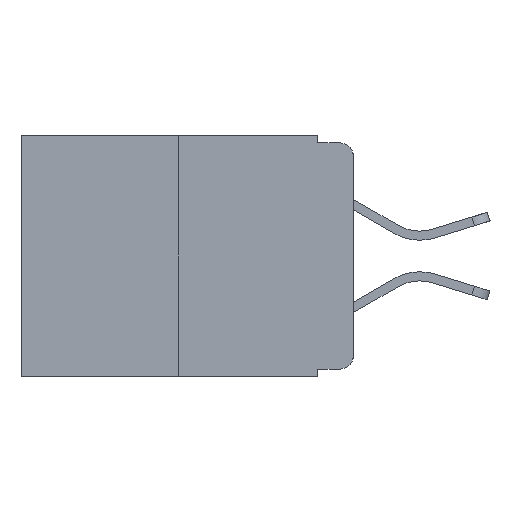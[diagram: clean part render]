
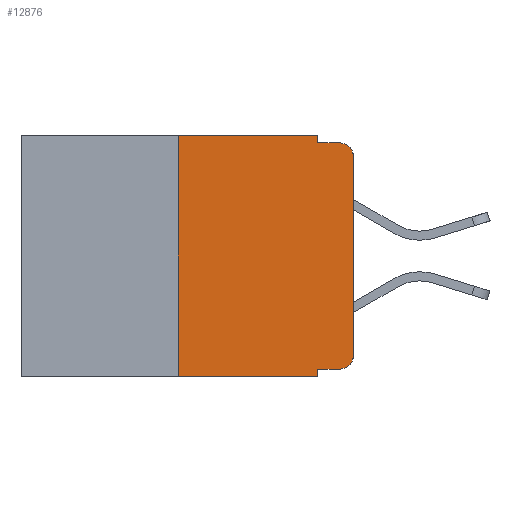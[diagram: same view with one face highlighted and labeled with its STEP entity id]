
A CAD part, left-side view. The second image highlights one B-rep face of the part: STEP entity #12876.
In plain terms, the highlighted planar face has unit normal (-1, 0, 0).
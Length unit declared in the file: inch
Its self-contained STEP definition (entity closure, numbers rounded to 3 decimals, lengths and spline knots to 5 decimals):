
#13 = DIRECTION ( 'NONE',  ( 0., 0., -1. ) ) ;
#335 = DIRECTION ( 'NONE',  ( 0., 0., -1. ) ) ;
#521 = VECTOR ( 'NONE', #4729, 39.37008 ) ;
#529 = CARTESIAN_POINT ( 'NONE',  ( 0., 0.051, -0.343 ) ) ;
#798 = LINE ( 'NONE', #15091, #11758 ) ;
#930 = LINE ( 'NONE', #16887, #11429 ) ;
#941 = CARTESIAN_POINT ( 'NONE',  ( 0., 0.25, 0. ) ) ;
#1084 = EDGE_CURVE ( 'NONE', #4803, #3712, #8154, .T. ) ;
#2283 = DIRECTION ( 'NONE',  ( -1., 0., 0. ) ) ;
#2502 = LINE ( 'NONE', #14109, #13431 ) ;
#2797 = CARTESIAN_POINT ( 'NONE',  ( 0., 0.473, 0. ) ) ;
#2988 = VERTEX_POINT ( 'NONE', #7426 ) ;
#3042 = EDGE_CURVE ( 'NONE', #4803, #16492, #13799, .T. ) ;
#3497 = CIRCLE ( 'NONE', #4543, 0.02 ) ;
#3712 = VERTEX_POINT ( 'NONE', #9028 ) ;
#4163 = CARTESIAN_POINT ( 'NONE',  ( 0., 0.02, -0.01 ) ) ;
#4246 = DIRECTION ( 'NONE',  ( 0., 0., -1. ) ) ;
#4267 = DIRECTION ( 'NONE',  ( 0., -1., 0. ) ) ;
#4543 = AXIS2_PLACEMENT_3D ( 'NONE', #8289, #17995, #9701 ) ;
#4729 = DIRECTION ( 'NONE',  ( 0., 0., 1. ) ) ;
#4803 = VERTEX_POINT ( 'NONE', #5604 ) ;
#4942 = ORIENTED_EDGE ( 'NONE', *, *, #16857, .T. ) ;
#4988 = EDGE_CURVE ( 'NONE', #12511, #10292, #11922, .T. ) ;
#5346 = LINE ( 'NONE', #14137, #6709 ) ;
#5362 = CARTESIAN_POINT ( 'NONE',  ( 0., 0.051, -0.01 ) ) ;
#5394 = ORIENTED_EDGE ( 'NONE', *, *, #1084, .T. ) ;
#5604 = CARTESIAN_POINT ( 'NONE',  ( 0., 0.051, -0.333 ) ) ;
#5852 = ORIENTED_EDGE ( 'NONE', *, *, #17550, .T. ) ;
#5960 = EDGE_CURVE ( 'NONE', #6591, #16915, #930, .T. ) ;
#6123 = CARTESIAN_POINT ( 'NONE',  ( 0., 0.051, 0. ) ) ;
#6591 = VERTEX_POINT ( 'NONE', #15372 ) ;
#6709 = VECTOR ( 'NONE', #15493, 39.37008 ) ;
#6919 = EDGE_CURVE ( 'NONE', #16915, #14463, #2502, .T. ) ;
#6967 = ORIENTED_EDGE ( 'NONE', *, *, #7891, .T. ) ;
#7372 = AXIS2_PLACEMENT_3D ( 'NONE', #16979, #8662, #13 ) ;
#7426 = CARTESIAN_POINT ( 'NONE',  ( 0., 0., -0.313 ) ) ;
#7873 = ORIENTED_EDGE ( 'NONE', *, *, #17674, .F. ) ;
#7891 = EDGE_CURVE ( 'NONE', #12473, #14463, #17437, .T. ) ;
#8154 = LINE ( 'NONE', #12954, #11407 ) ;
#8289 = CARTESIAN_POINT ( 'NONE',  ( 0., 0.02, -0.313 ) ) ;
#8318 = ORIENTED_EDGE ( 'NONE', *, *, #4988, .F. ) ;
#8662 = DIRECTION ( 'NONE',  ( 1., 0., 0. ) ) ;
#8828 = EDGE_CURVE ( 'NONE', #2988, #12473, #5346, .T. ) ;
#8903 = VECTOR ( 'NONE', #4267, 39.37008 ) ;
#9028 = CARTESIAN_POINT ( 'NONE',  ( 0., 0.02, -0.333 ) ) ;
#9175 = CARTESIAN_POINT ( 'NONE',  ( 0., 0., -0.03 ) ) ;
#9701 = DIRECTION ( 'NONE',  ( 0., 0., -1. ) ) ;
#10009 = PLANE ( 'NONE',  #7372 ) ;
#10060 = VECTOR ( 'NONE', #335, 39.37008 ) ;
#10142 = DIRECTION ( 'NONE',  ( 0., -1., 0. ) ) ;
#10292 = VERTEX_POINT ( 'NONE', #941 ) ;
#10375 = CARTESIAN_POINT ( 'NONE',  ( 0., 0.25, 0. ) ) ;
#10858 = CARTESIAN_POINT ( 'NONE',  ( 0., 0.02, -0.03 ) ) ;
#11131 = ORIENTED_EDGE ( 'NONE', *, *, #5960, .F. ) ;
#11407 = VECTOR ( 'NONE', #10142, 39.37008 ) ;
#11429 = VECTOR ( 'NONE', #4246, 39.37008 ) ;
#11758 = VECTOR ( 'NONE', #16448, 39.37008 ) ;
#11922 = LINE ( 'NONE', #10375, #521 ) ;
#12282 = DIRECTION ( 'NONE',  ( 0., 0., -1. ) ) ;
#12473 = VERTEX_POINT ( 'NONE', #9175 ) ;
#12480 = ORIENTED_EDGE ( 'NONE', *, *, #3042, .F. ) ;
#12511 = VERTEX_POINT ( 'NONE', #14859 ) ;
#12689 = DIRECTION ( 'NONE',  ( 0., -1., 0. ) ) ;
#12876 = ADVANCED_FACE ( 'NONE', ( #17888 ), #10009, .F. ) ;
#12954 = CARTESIAN_POINT ( 'NONE',  ( 0., 0.051, -0.333 ) ) ;
#13067 = LINE ( 'NONE', #2797, #8903 ) ;
#13431 = VECTOR ( 'NONE', #12689, 39.37008 ) ;
#13677 = EDGE_LOOP ( 'NONE', ( #14027, #6967, #14453, #11131, #7873, #8318, #4942, #12480, #5394, #5852 ) ) ;
#13799 = LINE ( 'NONE', #6123, #10060 ) ;
#14027 = ORIENTED_EDGE ( 'NONE', *, *, #8828, .T. ) ;
#14109 = CARTESIAN_POINT ( 'NONE',  ( 0., 0.051, -0.01 ) ) ;
#14137 = CARTESIAN_POINT ( 'NONE',  ( 0., 0., 0. ) ) ;
#14372 = AXIS2_PLACEMENT_3D ( 'NONE', #10858, #2283, #12282 ) ;
#14453 = ORIENTED_EDGE ( 'NONE', *, *, #6919, .F. ) ;
#14463 = VERTEX_POINT ( 'NONE', #4163 ) ;
#14859 = CARTESIAN_POINT ( 'NONE',  ( 0., 0.25, -0.343 ) ) ;
#15091 = CARTESIAN_POINT ( 'NONE',  ( 0., 0.473, -0.343 ) ) ;
#15372 = CARTESIAN_POINT ( 'NONE',  ( 0., 0.051, 0. ) ) ;
#15493 = DIRECTION ( 'NONE',  ( 0., 0., 1. ) ) ;
#16448 = DIRECTION ( 'NONE',  ( 0., -1., 0. ) ) ;
#16492 = VERTEX_POINT ( 'NONE', #529 ) ;
#16857 = EDGE_CURVE ( 'NONE', #12511, #16492, #798, .T. ) ;
#16887 = CARTESIAN_POINT ( 'NONE',  ( 0., 0.051, 0. ) ) ;
#16915 = VERTEX_POINT ( 'NONE', #5362 ) ;
#16979 = CARTESIAN_POINT ( 'NONE',  ( 0., 0.473, 0. ) ) ;
#17437 = CIRCLE ( 'NONE', #14372, 0.02 ) ;
#17550 = EDGE_CURVE ( 'NONE', #3712, #2988, #3497, .T. ) ;
#17674 = EDGE_CURVE ( 'NONE', #10292, #6591, #13067, .T. ) ;
#17888 = FACE_OUTER_BOUND ( 'NONE', #13677, .T. ) ;
#17995 = DIRECTION ( 'NONE',  ( -1., 0., 0. ) ) ;
